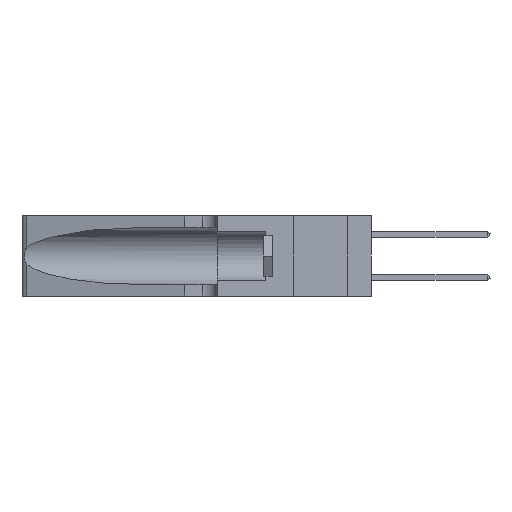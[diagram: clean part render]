
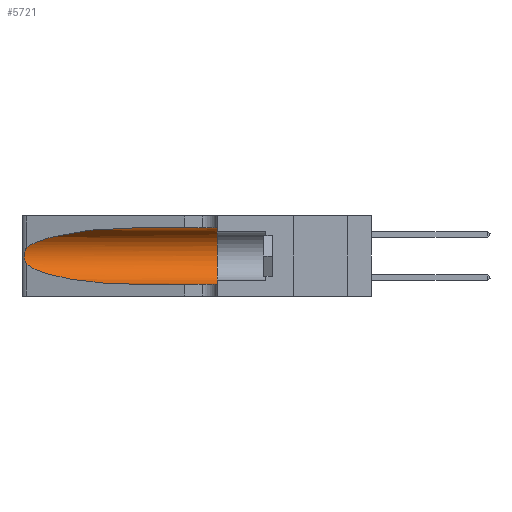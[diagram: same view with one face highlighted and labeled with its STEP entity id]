
A CAD part, left-side view. The second image highlights one B-rep face of the part: STEP entity #5721.
In plain terms, the highlighted cylindrical face has radius 3.308 mm (diameter 6.617 mm), a partial arc.
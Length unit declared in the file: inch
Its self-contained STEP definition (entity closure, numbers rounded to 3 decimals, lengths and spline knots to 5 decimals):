
#231 = VERTEX_POINT ( 'NONE', #5349 ) ;
#934 = VECTOR ( 'NONE', #3705, 39.37008 ) ;
#1214 = ORIENTED_EDGE ( 'NONE', *, *, #13673, .T. ) ;
#1966 = CARTESIAN_POINT ( 'NONE',  ( 0.25639, 1.23184, 0.21858 ) ) ;
#3035 = EDGE_LOOP ( 'NONE', ( #1214, #15226, #28191, #15700, #10417, #22960 ) ) ;
#3569 = CARTESIAN_POINT ( 'NONE',  ( 0.1305, 1.61858, 0.31525 ) ) ;
#3705 = DIRECTION ( 'NONE',  ( 0., -1., 0. ) ) ;
#5094 = EDGE_CURVE ( 'NONE', #7584, #29144, #16551, .T. ) ;
#5162 = CARTESIAN_POINT ( 'NONE',  ( 0.2373, 1.15595, 0.08982 ) ) ;
#5254 = VERTEX_POINT ( 'NONE', #12365 ) ;
#5349 = CARTESIAN_POINT ( 'NONE',  ( 0.1305, 0.35, 0.05475 ) ) ;
#5393 = VECTOR ( 'NONE', #10525, 39.37008 ) ;
#5590 = DIRECTION ( 'NONE',  ( 0., 0., -1. ) ) ;
#5721 = ADVANCED_FACE ( 'NONE', ( #28568 ), #22171, .F. ) ;
#5945 = CARTESIAN_POINT ( 'NONE',  ( 0.1305, 0.72297, 0.05475 ) ) ;
#6214 = CARTESIAN_POINT ( 'NONE',  ( 0.25789, 1.23486, 0.15765 ) ) ;
#6378 = CARTESIAN_POINT ( 'NONE',  ( 0.2373, 1.15595, 0.28018 ) ) ;
#6478 = CARTESIAN_POINT ( 'NONE',  ( 0.18966, 0.96281, 0.31525 ) ) ;
#6500 = CARTESIAN_POINT ( 'NONE',  ( 0.25854, 1.2359, 0.20912 ) ) ;
#7584 = VERTEX_POINT ( 'NONE', #26266 ) ;
#8775 = CARTESIAN_POINT ( 'NONE',  ( 0.26018, 1.23835, 0.19895 ) ) ;
#8977 = EDGE_CURVE ( 'NONE', #29144, #231, #13001, .T. ) ;
#9902 = CARTESIAN_POINT ( 'NONE',  ( 0.1305, 0.72297, 0.31525 ) ) ;
#10417 = ORIENTED_EDGE ( 'NONE', *, *, #22756, .F. ) ;
#10525 = DIRECTION ( 'NONE',  ( 0., -1., 0. ) ) ;
#10691 = CARTESIAN_POINT ( 'NONE',  ( 0.25787, 1.23484, 0.2124 ) ) ;
#11357 = EDGE_CURVE ( 'NONE', #14161, #17808, #11467, .T. ) ;
#11467 = LINE ( 'NONE', #3569, #5393 ) ;
#12365 = CARTESIAN_POINT ( 'NONE',  ( 0.25487, 1.22718, 0.22369 ) ) ;
#12724 = CARTESIAN_POINT ( 'NONE',  ( 0.18966, 0.96281, 0.05475 ) ) ;
#12991 = CARTESIAN_POINT ( 'NONE',  ( 0.26075, 1.23896, 0.178 ) ) ;
#13001 = LINE ( 'NONE', #26369, #934 ) ;
#13522 = B_SPLINE_CURVE_WITH_KNOTS ( 'NONE', 3,
 ( #17737, #19840, #1966, #10691, #6500, #8775, #24310, #12991, #28894, #17540, #6214, #22133, #26691, #15365 ),
 .UNSPECIFIED., .F., .F.,
 ( 4, 2, 2, 2, 2, 2, 4 ),
 ( 0., 0.00027, 0.00053, 0.00107, 0.0016, 0.00187, 0.00214 ),
 .UNSPECIFIED. ) ;
#13673 = EDGE_CURVE ( 'NONE', #14161, #5254, #20596, .T. ) ;
#13821 = AXIS2_PLACEMENT_3D ( 'NONE', #27113, #14470, #5590 ) ;
#14161 = VERTEX_POINT ( 'NONE', #9902 ) ;
#14470 = DIRECTION ( 'NONE',  ( 0., -1., 0. ) ) ;
#15157 = CARTESIAN_POINT ( 'NONE',  ( 0.25487, 1.22718, 0.22369 ) ) ;
#15226 = ORIENTED_EDGE ( 'NONE', *, *, #18760, .T. ) ;
#15323 = CARTESIAN_POINT ( 'NONE',  ( 0.1305, 0.72297, 0.05475 ) ) ;
#15365 = CARTESIAN_POINT ( 'NONE',  ( 0.25487, 1.22718, 0.14631 ) ) ;
#15700 = ORIENTED_EDGE ( 'NONE', *, *, #8977, .T. ) ;
#16551 =( BOUNDED_CURVE ( )  B_SPLINE_CURVE ( 3, ( #27377, #5162, #12724, #5945 ),
 .UNSPECIFIED., .F., .F. ) 
 B_SPLINE_CURVE_WITH_KNOTS ( ( 4, 4 ),
 ( 3.44316, 4.71239 ),
 .UNSPECIFIED. ) 
 CURVE ( )  GEOMETRIC_REPRESENTATION_ITEM ( )  RATIONAL_B_SPLINE_CURVE ( ( 1., 0.87, 0.87, 1. ) ) 
 REPRESENTATION_ITEM ( '' )  );
#17540 = CARTESIAN_POINT ( 'NONE',  ( 0.25856, 1.23593, 0.16098 ) ) ;
#17627 = CIRCLE ( 'NONE', #25680, 0.13025 ) ;
#17737 = CARTESIAN_POINT ( 'NONE',  ( 0.25487, 1.22718, 0.22369 ) ) ;
#17808 = VERTEX_POINT ( 'NONE', #17814 ) ;
#17814 = CARTESIAN_POINT ( 'NONE',  ( 0.1305, 0.35, 0.31525 ) ) ;
#18760 = EDGE_CURVE ( 'NONE', #5254, #7584, #13522, .T. ) ;
#19597 = CARTESIAN_POINT ( 'NONE',  ( 0.1305, 0.35, 0.185 ) ) ;
#19840 = CARTESIAN_POINT ( 'NONE',  ( 0.25555, 1.22994, 0.2215 ) ) ;
#20596 =( BOUNDED_CURVE ( )  B_SPLINE_CURVE ( 3, ( #29075, #6478, #6378, #15157 ),
 .UNSPECIFIED., .F., .T. ) 
 B_SPLINE_CURVE_WITH_KNOTS ( ( 4, 4 ),
 ( 1.5708, 2.84003 ),
 .UNSPECIFIED. ) 
 CURVE ( )  GEOMETRIC_REPRESENTATION_ITEM ( )  RATIONAL_B_SPLINE_CURVE ( ( 1., 0.87, 0.87, 1. ) ) 
 REPRESENTATION_ITEM ( '' )  );
#21895 = DIRECTION ( 'NONE',  ( 0., 1., 0. ) ) ;
#22133 = CARTESIAN_POINT ( 'NONE',  ( 0.25639, 1.23186, 0.15144 ) ) ;
#22171 = CYLINDRICAL_SURFACE ( 'NONE', #13821, 0.13025 ) ;
#22756 = EDGE_CURVE ( 'NONE', #17808, #231, #17627, .T. ) ;
#22960 = ORIENTED_EDGE ( 'NONE', *, *, #11357, .F. ) ;
#24310 = CARTESIAN_POINT ( 'NONE',  ( 0.26075, 1.23896, 0.19203 ) ) ;
#25680 = AXIS2_PLACEMENT_3D ( 'NONE', #19597, #21895, #26457 ) ;
#26266 = CARTESIAN_POINT ( 'NONE',  ( 0.25487, 1.22718, 0.14631 ) ) ;
#26369 = CARTESIAN_POINT ( 'NONE',  ( 0.1305, 1.61858, 0.05475 ) ) ;
#26457 = DIRECTION ( 'NONE',  ( 0., 0., 1. ) ) ;
#26691 = CARTESIAN_POINT ( 'NONE',  ( 0.25555, 1.22993, 0.14849 ) ) ;
#27113 = CARTESIAN_POINT ( 'NONE',  ( 0.1305, 1.61858, 0.185 ) ) ;
#27377 = CARTESIAN_POINT ( 'NONE',  ( 0.25487, 1.22718, 0.14631 ) ) ;
#28191 = ORIENTED_EDGE ( 'NONE', *, *, #5094, .T. ) ;
#28568 = FACE_OUTER_BOUND ( 'NONE', #3035, .T. ) ;
#28894 = CARTESIAN_POINT ( 'NONE',  ( 0.26017, 1.23833, 0.17102 ) ) ;
#29075 = CARTESIAN_POINT ( 'NONE',  ( 0.1305, 0.72297, 0.31525 ) ) ;
#29144 = VERTEX_POINT ( 'NONE', #15323 ) ;
